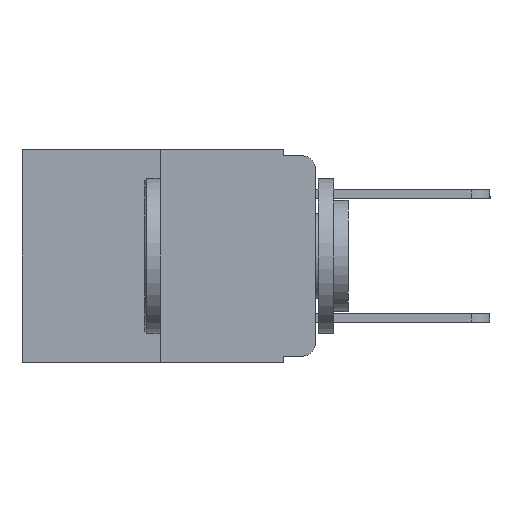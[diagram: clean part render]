
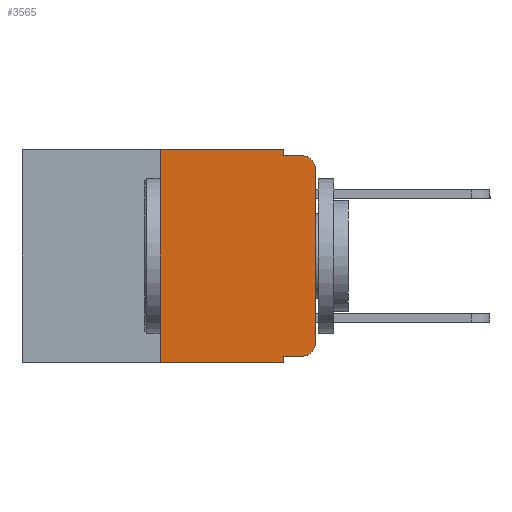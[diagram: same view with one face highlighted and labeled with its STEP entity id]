
A CAD part, left-side view. The second image highlights one B-rep face of the part: STEP entity #3565.
In plain terms, the highlighted planar face has unit normal (-1, 0, 0).
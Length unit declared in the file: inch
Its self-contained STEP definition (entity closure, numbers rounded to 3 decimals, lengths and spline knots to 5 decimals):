
#111 = VERTEX_POINT ( 'NONE', #10271 ) ;
#183 = VERTEX_POINT ( 'NONE', #8803 ) ;
#506 = CARTESIAN_POINT ( 'NONE',  ( 0., 0.051, -0.01 ) ) ;
#668 = LINE ( 'NONE', #506, #5140 ) ;
#905 = EDGE_CURVE ( 'NONE', #183, #6413, #10188, .T. ) ;
#1229 = CARTESIAN_POINT ( 'NONE',  ( 0., 0., -0.313 ) ) ;
#1413 = DIRECTION ( 'NONE',  ( 0., -1., 0. ) ) ;
#1479 = LINE ( 'NONE', #9536, #9824 ) ;
#1747 = FACE_OUTER_BOUND ( 'NONE', #4113, .T. ) ;
#2002 = VERTEX_POINT ( 'NONE', #5791 ) ;
#2221 = VERTEX_POINT ( 'NONE', #8833 ) ;
#2247 = ORIENTED_EDGE ( 'NONE', *, *, #10362, .T. ) ;
#2248 = AXIS2_PLACEMENT_3D ( 'NONE', #2851, #4151, #3712 ) ;
#2373 = CARTESIAN_POINT ( 'NONE',  ( 0., 0.02, -0.313 ) ) ;
#2417 = LINE ( 'NONE', #9576, #8661 ) ;
#2456 = EDGE_CURVE ( 'NONE', #4740, #111, #6706, .T. ) ;
#2506 = CARTESIAN_POINT ( 'NONE',  ( 0., 0.051, 0. ) ) ;
#2585 = ORIENTED_EDGE ( 'NONE', *, *, #2456, .T. ) ;
#2760 = CARTESIAN_POINT ( 'NONE',  ( 0., 0.051, 0. ) ) ;
#2851 = CARTESIAN_POINT ( 'NONE',  ( 0., 0.473, 0. ) ) ;
#2898 = EDGE_CURVE ( 'NONE', #3044, #4771, #10150, .T. ) ;
#2942 = ORIENTED_EDGE ( 'NONE', *, *, #9619, .F. ) ;
#3041 = DIRECTION ( 'NONE',  ( 0., 0., -1. ) ) ;
#3044 = VERTEX_POINT ( 'NONE', #9688 ) ;
#3148 = CIRCLE ( 'NONE', #9482, 0.02 ) ;
#3253 = ORIENTED_EDGE ( 'NONE', *, *, #3298, .F. ) ;
#3298 = EDGE_CURVE ( 'NONE', #4771, #3420, #4573, .T. ) ;
#3394 = CARTESIAN_POINT ( 'NONE',  ( 0., 0.051, 0. ) ) ;
#3420 = VERTEX_POINT ( 'NONE', #6947 ) ;
#3551 = ORIENTED_EDGE ( 'NONE', *, *, #2898, .F. ) ;
#3565 = ADVANCED_FACE ( 'NONE', ( #1747 ), #5951, .F. ) ;
#3712 = DIRECTION ( 'NONE',  ( 0., 0., -1. ) ) ;
#3713 = ORIENTED_EDGE ( 'NONE', *, *, #10249, .F. ) ;
#3734 = CARTESIAN_POINT ( 'NONE',  ( 0., 0.473, -0.343 ) ) ;
#3948 = ORIENTED_EDGE ( 'NONE', *, *, #905, .T. ) ;
#4113 = EDGE_LOOP ( 'NONE', ( #2247, #2585, #2942, #3253, #3551, #3713, #3948, #4236, #4254, #4508 ) ) ;
#4151 = DIRECTION ( 'NONE',  ( 1., 0., 0. ) ) ;
#4236 = ORIENTED_EDGE ( 'NONE', *, *, #5792, .F. ) ;
#4254 = ORIENTED_EDGE ( 'NONE', *, *, #7531, .T. ) ;
#4508 = ORIENTED_EDGE ( 'NONE', *, *, #5454, .T. ) ;
#4573 = LINE ( 'NONE', #2506, #8476 ) ;
#4740 = VERTEX_POINT ( 'NONE', #5372 ) ;
#4771 = VERTEX_POINT ( 'NONE', #2760 ) ;
#4807 = DIRECTION ( 'NONE',  ( -1., 0., 0. ) ) ;
#4825 = DIRECTION ( 'NONE',  ( 0., 0., -1. ) ) ;
#4979 = LINE ( 'NONE', #6404, #9728 ) ;
#4983 = DIRECTION ( 'NONE',  ( 0., 0., 1. ) ) ;
#5140 = VECTOR ( 'NONE', #1413, 39.37008 ) ;
#5372 = CARTESIAN_POINT ( 'NONE',  ( 0., 0., -0.03 ) ) ;
#5454 = EDGE_CURVE ( 'NONE', #2002, #6934, #3148, .T. ) ;
#5530 = CARTESIAN_POINT ( 'NONE',  ( 0., 0.051, -0.343 ) ) ;
#5791 = CARTESIAN_POINT ( 'NONE',  ( 0., 0.02, -0.333 ) ) ;
#5792 = EDGE_CURVE ( 'NONE', #2221, #6413, #9894, .T. ) ;
#5872 = DIRECTION ( 'NONE',  ( -1., 0., 0. ) ) ;
#5939 = VECTOR ( 'NONE', #7574, 39.37008 ) ;
#5951 = PLANE ( 'NONE',  #2248 ) ;
#6202 = VECTOR ( 'NONE', #7485, 39.37008 ) ;
#6404 = CARTESIAN_POINT ( 'NONE',  ( 0., 0.25, 0. ) ) ;
#6413 = VERTEX_POINT ( 'NONE', #5530 ) ;
#6706 = CIRCLE ( 'NONE', #8422, 0.02 ) ;
#6934 = VERTEX_POINT ( 'NONE', #1229 ) ;
#6947 = CARTESIAN_POINT ( 'NONE',  ( 0., 0.051, -0.01 ) ) ;
#7208 = CARTESIAN_POINT ( 'NONE',  ( 0., 0.02, -0.03 ) ) ;
#7485 = DIRECTION ( 'NONE',  ( 0., -1., 0. ) ) ;
#7531 = EDGE_CURVE ( 'NONE', #2221, #2002, #2417, .T. ) ;
#7574 = DIRECTION ( 'NONE',  ( 0., 0., -1. ) ) ;
#8303 = VECTOR ( 'NONE', #8776, 39.37008 ) ;
#8422 = AXIS2_PLACEMENT_3D ( 'NONE', #7208, #5872, #4825 ) ;
#8462 = DIRECTION ( 'NONE',  ( 0., -1., 0. ) ) ;
#8476 = VECTOR ( 'NONE', #9919, 39.37008 ) ;
#8661 = VECTOR ( 'NONE', #8462, 39.37008 ) ;
#8776 = DIRECTION ( 'NONE',  ( 0., -1., 0. ) ) ;
#8803 = CARTESIAN_POINT ( 'NONE',  ( 0., 0.25, -0.343 ) ) ;
#8833 = CARTESIAN_POINT ( 'NONE',  ( 0., 0.051, -0.333 ) ) ;
#9417 = DIRECTION ( 'NONE',  ( 0., 0., 1. ) ) ;
#9482 = AXIS2_PLACEMENT_3D ( 'NONE', #2373, #4807, #3041 ) ;
#9536 = CARTESIAN_POINT ( 'NONE',  ( 0., 0., 0. ) ) ;
#9576 = CARTESIAN_POINT ( 'NONE',  ( 0., 0.051, -0.333 ) ) ;
#9619 = EDGE_CURVE ( 'NONE', #3420, #111, #668, .T. ) ;
#9688 = CARTESIAN_POINT ( 'NONE',  ( 0., 0.25, 0. ) ) ;
#9728 = VECTOR ( 'NONE', #9417, 39.37008 ) ;
#9824 = VECTOR ( 'NONE', #4983, 39.37008 ) ;
#9894 = LINE ( 'NONE', #3394, #5939 ) ;
#9919 = DIRECTION ( 'NONE',  ( 0., 0., -1. ) ) ;
#10150 = LINE ( 'NONE', #10204, #6202 ) ;
#10188 = LINE ( 'NONE', #3734, #8303 ) ;
#10204 = CARTESIAN_POINT ( 'NONE',  ( 0., 0.473, 0. ) ) ;
#10249 = EDGE_CURVE ( 'NONE', #183, #3044, #4979, .T. ) ;
#10271 = CARTESIAN_POINT ( 'NONE',  ( 0., 0.02, -0.01 ) ) ;
#10362 = EDGE_CURVE ( 'NONE', #6934, #4740, #1479, .T. ) ;
